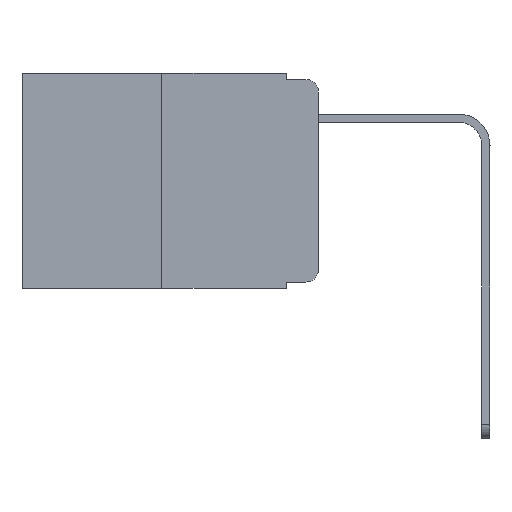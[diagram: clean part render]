
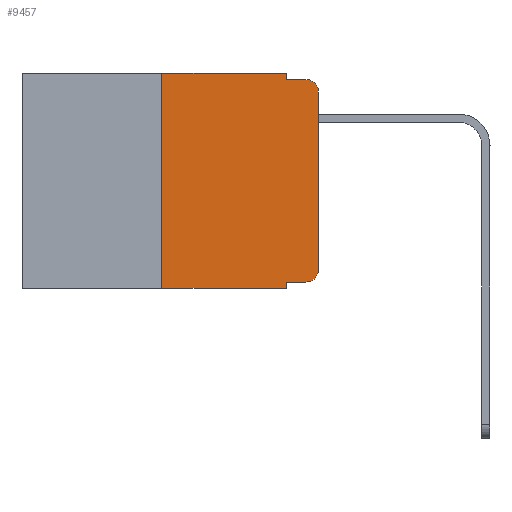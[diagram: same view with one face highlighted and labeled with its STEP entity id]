
A CAD part, left-side view. The second image highlights one B-rep face of the part: STEP entity #9457.
In plain terms, the highlighted planar face has unit normal (-1, 0, 0).
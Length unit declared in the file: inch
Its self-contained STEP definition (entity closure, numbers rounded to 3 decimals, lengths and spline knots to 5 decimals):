
#93 = VERTEX_POINT ( 'NONE', #12762 ) ;
#427 = CARTESIAN_POINT ( 'NONE',  ( 0., 0.25, -0.343 ) ) ;
#585 = VERTEX_POINT ( 'NONE', #4426 ) ;
#1305 = DIRECTION ( 'NONE',  ( 0., -1., 0. ) ) ;
#1365 = VECTOR ( 'NONE', #4780, 39.37008 ) ;
#1658 = CARTESIAN_POINT ( 'NONE',  ( 0., 0.473, 0. ) ) ;
#1950 = VECTOR ( 'NONE', #7397, 39.37008 ) ;
#1990 = AXIS2_PLACEMENT_3D ( 'NONE', #9561, #2167, #4718 ) ;
#2074 = CARTESIAN_POINT ( 'NONE',  ( 0., 0.051, -0.01 ) ) ;
#2148 = ORIENTED_EDGE ( 'NONE', *, *, #15050, .T. ) ;
#2167 = DIRECTION ( 'NONE',  ( -1., 0., 0. ) ) ;
#2210 = VERTEX_POINT ( 'NONE', #13949 ) ;
#2316 = LINE ( 'NONE', #14673, #1365 ) ;
#2730 = DIRECTION ( 'NONE',  ( 0., 0., -1. ) ) ;
#2885 = VECTOR ( 'NONE', #1305, 39.37008 ) ;
#2909 = ORIENTED_EDGE ( 'NONE', *, *, #7279, .T. ) ;
#3183 = CARTESIAN_POINT ( 'NONE',  ( 0., 0.051, -0.333 ) ) ;
#3278 = EDGE_CURVE ( 'NONE', #11766, #93, #14907, .T. ) ;
#3600 = VERTEX_POINT ( 'NONE', #6495 ) ;
#3893 = EDGE_CURVE ( 'NONE', #11287, #3600, #12011, .T. ) ;
#3977 = VECTOR ( 'NONE', #15221, 39.37008 ) ;
#4120 = ORIENTED_EDGE ( 'NONE', *, *, #12375, .T. ) ;
#4426 = CARTESIAN_POINT ( 'NONE',  ( 0., 0.051, -0.343 ) ) ;
#4718 = DIRECTION ( 'NONE',  ( 0., 0., -1. ) ) ;
#4780 = DIRECTION ( 'NONE',  ( 0., 0., -1. ) ) ;
#4794 = AXIS2_PLACEMENT_3D ( 'NONE', #1658, #10133, #2730 ) ;
#4920 = CARTESIAN_POINT ( 'NONE',  ( 0., 0.051, -0.333 ) ) ;
#5612 = DIRECTION ( 'NONE',  ( 0., -1., 0. ) ) ;
#6412 = VECTOR ( 'NONE', #14129, 39.37008 ) ;
#6495 = CARTESIAN_POINT ( 'NONE',  ( 0., 0.02, -0.01 ) ) ;
#6571 = VECTOR ( 'NONE', #8143, 39.37008 ) ;
#6700 = CARTESIAN_POINT ( 'NONE',  ( 0., 0., -0.03 ) ) ;
#6848 = CARTESIAN_POINT ( 'NONE',  ( 0., 0.051, -0.01 ) ) ;
#6968 = DIRECTION ( 'NONE',  ( 0., 0., -1. ) ) ;
#7279 = EDGE_CURVE ( 'NONE', #12451, #2210, #14299, .T. ) ;
#7397 = DIRECTION ( 'NONE',  ( 0., -1., 0. ) ) ;
#7433 = CARTESIAN_POINT ( 'NONE',  ( 0., 0.473, 0. ) ) ;
#7440 = ORIENTED_EDGE ( 'NONE', *, *, #8043, .F. ) ;
#7583 = EDGE_CURVE ( 'NONE', #12451, #585, #11586, .T. ) ;
#7792 = EDGE_CURVE ( 'NONE', #8463, #3600, #11994, .T. ) ;
#7843 = LINE ( 'NONE', #11364, #3977 ) ;
#7891 = LINE ( 'NONE', #7433, #2885 ) ;
#8043 = EDGE_CURVE ( 'NONE', #93, #13715, #7891, .T. ) ;
#8143 = DIRECTION ( 'NONE',  ( 0., 0., 1. ) ) ;
#8184 = DIRECTION ( 'NONE',  ( -1., 0., 0. ) ) ;
#8210 = CARTESIAN_POINT ( 'NONE',  ( 0., 0.051, 0. ) ) ;
#8463 = VERTEX_POINT ( 'NONE', #2074 ) ;
#9046 = PLANE ( 'NONE',  #4794 ) ;
#9411 = EDGE_CURVE ( 'NONE', #15768, #11287, #7843, .T. ) ;
#9457 = ADVANCED_FACE ( 'NONE', ( #12884 ), #9046, .F. ) ;
#9561 = CARTESIAN_POINT ( 'NONE',  ( 0., 0.02, -0.03 ) ) ;
#9622 = ORIENTED_EDGE ( 'NONE', *, *, #3278, .F. ) ;
#9662 = VECTOR ( 'NONE', #5612, 39.37008 ) ;
#9739 = CARTESIAN_POINT ( 'NONE',  ( 0., 0., -0.313 ) ) ;
#10133 = DIRECTION ( 'NONE',  ( 1., 0., 0. ) ) ;
#10187 = ORIENTED_EDGE ( 'NONE', *, *, #9411, .T. ) ;
#10449 = DIRECTION ( 'NONE',  ( 0., 0., -1. ) ) ;
#10563 = ORIENTED_EDGE ( 'NONE', *, *, #7792, .F. ) ;
#10964 = EDGE_LOOP ( 'NONE', ( #10187, #11359, #10563, #14133, #7440, #9622, #4120, #13682, #2909, #2148 ) ) ;
#11287 = VERTEX_POINT ( 'NONE', #6700 ) ;
#11359 = ORIENTED_EDGE ( 'NONE', *, *, #3893, .T. ) ;
#11364 = CARTESIAN_POINT ( 'NONE',  ( 0., 0., 0. ) ) ;
#11586 = LINE ( 'NONE', #14056, #13338 ) ;
#11658 = LINE ( 'NONE', #12959, #6412 ) ;
#11766 = VERTEX_POINT ( 'NONE', #427 ) ;
#11994 = LINE ( 'NONE', #6848, #9662 ) ;
#12011 = CIRCLE ( 'NONE', #1990, 0.02 ) ;
#12375 = EDGE_CURVE ( 'NONE', #11766, #585, #11658, .T. ) ;
#12451 = VERTEX_POINT ( 'NONE', #3183 ) ;
#12762 = CARTESIAN_POINT ( 'NONE',  ( 0., 0.25, 0. ) ) ;
#12884 = FACE_OUTER_BOUND ( 'NONE', #10964, .T. ) ;
#12959 = CARTESIAN_POINT ( 'NONE',  ( 0., 0.473, -0.343 ) ) ;
#13057 = CARTESIAN_POINT ( 'NONE',  ( 0., 0.02, -0.313 ) ) ;
#13072 = CARTESIAN_POINT ( 'NONE',  ( 0., 0.25, 0. ) ) ;
#13338 = VECTOR ( 'NONE', #10449, 39.37008 ) ;
#13682 = ORIENTED_EDGE ( 'NONE', *, *, #7583, .F. ) ;
#13715 = VERTEX_POINT ( 'NONE', #8210 ) ;
#13949 = CARTESIAN_POINT ( 'NONE',  ( 0., 0.02, -0.333 ) ) ;
#14056 = CARTESIAN_POINT ( 'NONE',  ( 0., 0.051, 0. ) ) ;
#14129 = DIRECTION ( 'NONE',  ( 0., -1., 0. ) ) ;
#14133 = ORIENTED_EDGE ( 'NONE', *, *, #14658, .F. ) ;
#14299 = LINE ( 'NONE', #4920, #1950 ) ;
#14658 = EDGE_CURVE ( 'NONE', #13715, #8463, #2316, .T. ) ;
#14673 = CARTESIAN_POINT ( 'NONE',  ( 0., 0.051, 0. ) ) ;
#14907 = LINE ( 'NONE', #13072, #6571 ) ;
#15050 = EDGE_CURVE ( 'NONE', #2210, #15768, #15678, .T. ) ;
#15221 = DIRECTION ( 'NONE',  ( 0., 0., 1. ) ) ;
#15239 = AXIS2_PLACEMENT_3D ( 'NONE', #13057, #8184, #6968 ) ;
#15678 = CIRCLE ( 'NONE', #15239, 0.02 ) ;
#15768 = VERTEX_POINT ( 'NONE', #9739 ) ;
